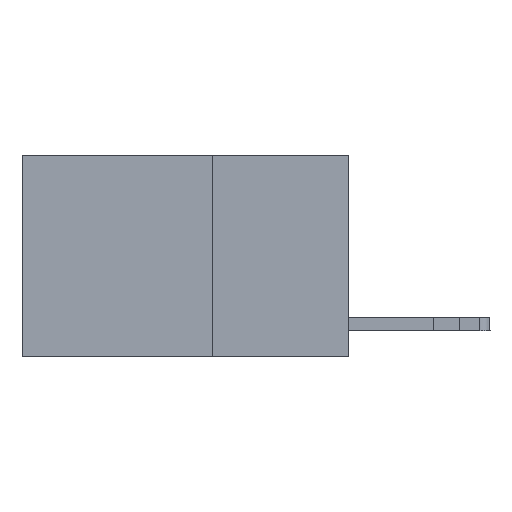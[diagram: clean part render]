
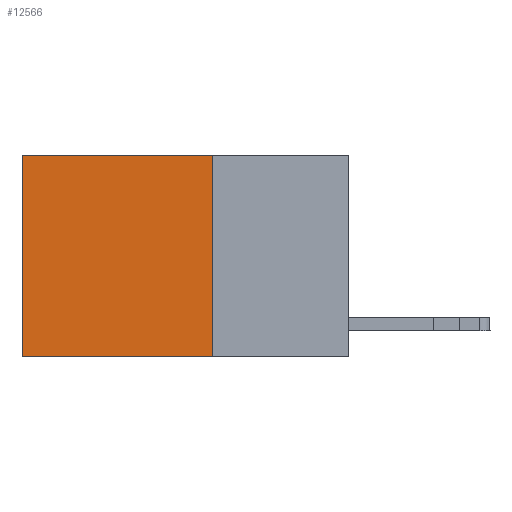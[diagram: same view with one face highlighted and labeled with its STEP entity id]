
A CAD part, left-side view. The second image highlights one B-rep face of the part: STEP entity #12566.
In plain terms, the highlighted planar face has unit normal (-1, 0, 0).
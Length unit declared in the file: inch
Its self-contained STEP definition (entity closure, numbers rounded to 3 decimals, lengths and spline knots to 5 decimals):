
#575 = VERTEX_POINT ( 'NONE', #22316 ) ;
#823 = ORIENTED_EDGE ( 'NONE', *, *, #19679, .F. ) ;
#1168 = ORIENTED_EDGE ( 'NONE', *, *, #12386, .F. ) ;
#1321 = LINE ( 'NONE', #9568, #16406 ) ;
#1367 = VERTEX_POINT ( 'NONE', #14985 ) ;
#2655 = CARTESIAN_POINT ( 'NONE',  ( 0.2625, 0.6, 0. ) ) ;
#3193 = EDGE_LOOP ( 'NONE', ( #4717, #823, #1168, #9996 ) ) ;
#3411 = CARTESIAN_POINT ( 'NONE',  ( 0.2625, 0.25, 0. ) ) ;
#3523 = FACE_OUTER_BOUND ( 'NONE', #3193, .T. ) ;
#4717 = ORIENTED_EDGE ( 'NONE', *, *, #19439, .T. ) ;
#6719 = DIRECTION ( 'NONE',  ( 0., 1., 0. ) ) ;
#8422 = LINE ( 'NONE', #15487, #20474 ) ;
#8551 = LINE ( 'NONE', #11930, #9025 ) ;
#9025 = VECTOR ( 'NONE', #6719, 39.37008 ) ;
#9568 = CARTESIAN_POINT ( 'NONE',  ( 0.2625, 0.25, 0. ) ) ;
#9996 = ORIENTED_EDGE ( 'NONE', *, *, #18158, .T. ) ;
#11248 = AXIS2_PLACEMENT_3D ( 'NONE', #3411, #17488, #19326 ) ;
#11252 = VERTEX_POINT ( 'NONE', #15531 ) ;
#11551 = LINE ( 'NONE', #2655, #14949 ) ;
#11799 = DIRECTION ( 'NONE',  ( 0., 0., -1. ) ) ;
#11930 = CARTESIAN_POINT ( 'NONE',  ( 0.2625, 0.25, 0. ) ) ;
#12386 = EDGE_CURVE ( 'NONE', #1367, #20462, #1321, .T. ) ;
#12566 = ADVANCED_FACE ( 'NONE', ( #3523 ), #17607, .F. ) ;
#14871 = DIRECTION ( 'NONE',  ( 0., 0., -1. ) ) ;
#14949 = VECTOR ( 'NONE', #11799, 39.37008 ) ;
#14985 = CARTESIAN_POINT ( 'NONE',  ( 0.2625, 0.25, 0. ) ) ;
#15487 = CARTESIAN_POINT ( 'NONE',  ( 0.2625, 0.25, -0.37 ) ) ;
#15531 = CARTESIAN_POINT ( 'NONE',  ( 0.2625, 0.6, -0.37 ) ) ;
#16406 = VECTOR ( 'NONE', #14871, 39.37008 ) ;
#17488 = DIRECTION ( 'NONE',  ( 1., 0., 0. ) ) ;
#17607 = PLANE ( 'NONE',  #11248 ) ;
#18158 = EDGE_CURVE ( 'NONE', #1367, #575, #8551, .T. ) ;
#18879 = CARTESIAN_POINT ( 'NONE',  ( 0.2625, 0.25, -0.37 ) ) ;
#19326 = DIRECTION ( 'NONE',  ( 0., 0., -1. ) ) ;
#19439 = EDGE_CURVE ( 'NONE', #575, #11252, #11551, .T. ) ;
#19679 = EDGE_CURVE ( 'NONE', #20462, #11252, #8422, .T. ) ;
#20462 = VERTEX_POINT ( 'NONE', #18879 ) ;
#20474 = VECTOR ( 'NONE', #22526, 39.37008 ) ;
#22316 = CARTESIAN_POINT ( 'NONE',  ( 0.2625, 0.6, 0. ) ) ;
#22526 = DIRECTION ( 'NONE',  ( 0., 1., 0. ) ) ;
